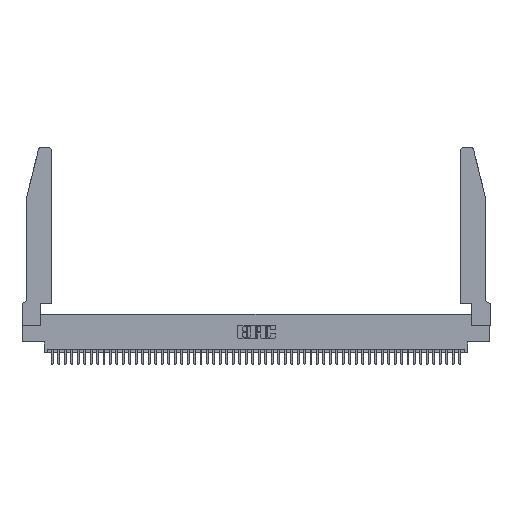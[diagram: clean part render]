
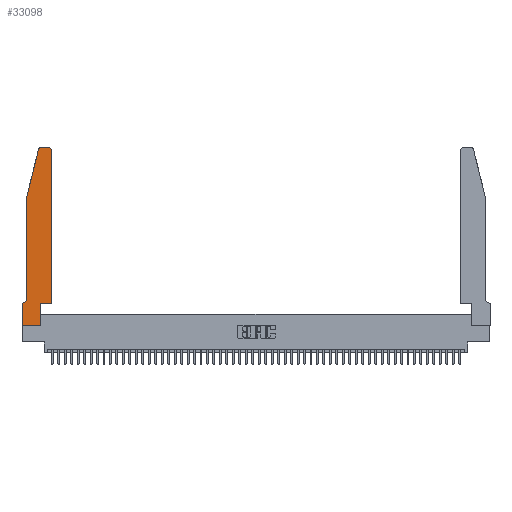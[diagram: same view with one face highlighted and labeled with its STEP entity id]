
A CAD part, top view. The second image highlights one B-rep face of the part: STEP entity #33098.
In plain terms, the highlighted planar face has unit normal (0, 0, 1).
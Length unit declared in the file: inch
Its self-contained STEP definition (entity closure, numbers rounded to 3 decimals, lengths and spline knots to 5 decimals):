
#779 = CARTESIAN_POINT ( 'NONE',  ( 0.4505, 0.35, 0.37 ) ) ;
#1848 = VECTOR ( 'NONE', #27411, 39.37008 ) ;
#1959 = EDGE_CURVE ( 'NONE', #48809, #43908, #16436, .T. ) ;
#2131 = DIRECTION ( 'NONE',  ( 1., 0., 0. ) ) ;
#2975 = ORIENTED_EDGE ( 'NONE', *, *, #28512, .T. ) ;
#3312 = CARTESIAN_POINT ( 'NONE',  ( 0., 0., 0.37 ) ) ;
#3450 = EDGE_CURVE ( 'NONE', #4753, #48809, #9399, .T. ) ;
#3521 = CARTESIAN_POINT ( 'NONE',  ( 0.0755, 2., 0.37 ) ) ;
#4753 = VERTEX_POINT ( 'NONE', #40390 ) ;
#4841 = CARTESIAN_POINT ( 'NONE',  ( 0.0755, 2., 0.37 ) ) ;
#5191 = LINE ( 'NONE', #779, #24251 ) ;
#6237 = EDGE_CURVE ( 'NONE', #11173, #46021, #50809, .T. ) ;
#6411 = VECTOR ( 'NONE', #9913, 39.37008 ) ;
#7217 = EDGE_CURVE ( 'NONE', #46886, #4753, #5191, .T. ) ;
#8631 = EDGE_CURVE ( 'NONE', #9656, #9747, #49717, .T. ) ;
#9015 = ORIENTED_EDGE ( 'NONE', *, *, #6237, .T. ) ;
#9399 = LINE ( 'NONE', #51511, #1848 ) ;
#9656 = VERTEX_POINT ( 'NONE', #24666 ) ;
#9747 = VERTEX_POINT ( 'NONE', #34577 ) ;
#9913 = DIRECTION ( 'NONE',  ( -1., 0., 0. ) ) ;
#10000 = CARTESIAN_POINT ( 'NONE',  ( 0.284, 2.72, 0.37 ) ) ;
#10002 = CARTESIAN_POINT ( 'NONE',  ( 0., 0.35, 0.37 ) ) ;
#11173 = VERTEX_POINT ( 'NONE', #37242 ) ;
#12496 = VECTOR ( 'NONE', #22220, 39.37008 ) ;
#13555 = ORIENTED_EDGE ( 'NONE', *, *, #1959, .T. ) ;
#14165 = DIRECTION ( 'NONE',  ( 1., 0., 0. ) ) ;
#15088 = ORIENTED_EDGE ( 'NONE', *, *, #28215, .T. ) ;
#15127 = ORIENTED_EDGE ( 'NONE', *, *, #3450, .T. ) ;
#16436 = CIRCLE ( 'NONE', #22639, 0.03 ) ;
#16842 = DIRECTION ( 'NONE',  ( 1., 0., 0. ) ) ;
#18253 = PLANE ( 'NONE',  #43515 ) ;
#18299 = VECTOR ( 'NONE', #2131, 39.37008 ) ;
#19898 = ORIENTED_EDGE ( 'NONE', *, *, #36210, .T. ) ;
#20077 = CARTESIAN_POINT ( 'NONE',  ( 0.2865, 0., 0.37 ) ) ;
#21431 = CARTESIAN_POINT ( 'NONE',  ( 0.4505, 2.72, 0.37 ) ) ;
#22161 = DIRECTION ( 'NONE',  ( 0., 0., 1. ) ) ;
#22216 = DIRECTION ( 'NONE',  ( 1., 0., 0. ) ) ;
#22220 = DIRECTION ( 'NONE',  ( 0., -1., 0. ) ) ;
#22243 = DIRECTION ( 'NONE',  ( -1., 0., 0. ) ) ;
#22639 = AXIS2_PLACEMENT_3D ( 'NONE', #30525, #38760, #26486 ) ;
#22997 = VECTOR ( 'NONE', #37019, 39.37008 ) ;
#23405 = DIRECTION ( 'NONE',  ( 0., -1., 0. ) ) ;
#23525 = LINE ( 'NONE', #3521, #24795 ) ;
#23817 = AXIS2_PLACEMENT_3D ( 'NONE', #10000, #38092, #22216 ) ;
#24251 = VECTOR ( 'NONE', #16842, 39.37008 ) ;
#24666 = CARTESIAN_POINT ( 'NONE',  ( 0.284, 2.75, 0.37 ) ) ;
#24795 = VECTOR ( 'NONE', #23405, 39.37008 ) ;
#25742 = CARTESIAN_POINT ( 'NONE',  ( 0., 0.35, 0.37 ) ) ;
#25931 = ORIENTED_EDGE ( 'NONE', *, *, #41141, .T. ) ;
#26433 = CARTESIAN_POINT ( 'NONE',  ( 0., 0., 0.37 ) ) ;
#26486 = DIRECTION ( 'NONE',  ( 1., 0., 0. ) ) ;
#26749 = DIRECTION ( 'NONE',  ( -1., 0., 0. ) ) ;
#26889 = EDGE_CURVE ( 'NONE', #9747, #51867, #27565, .T. ) ;
#27031 = VECTOR ( 'NONE', #37364, 39.37008 ) ;
#27411 = DIRECTION ( 'NONE',  ( 0., 1., 0. ) ) ;
#27565 = LINE ( 'NONE', #4841, #22997 ) ;
#28215 = EDGE_CURVE ( 'NONE', #43908, #9656, #31769, .T. ) ;
#28512 = EDGE_CURVE ( 'NONE', #51867, #11173, #23525, .T. ) ;
#30525 = CARTESIAN_POINT ( 'NONE',  ( 0.4205, 2.72, 0.37 ) ) ;
#30794 = ORIENTED_EDGE ( 'NONE', *, *, #8631, .T. ) ;
#30974 = LINE ( 'NONE', #26433, #18299 ) ;
#30993 = CARTESIAN_POINT ( 'NONE',  ( 0.4205, 2.75, 0.37 ) ) ;
#31046 = VERTEX_POINT ( 'NONE', #10002 ) ;
#31369 = FACE_OUTER_BOUND ( 'NONE', #48985, .T. ) ;
#31769 = LINE ( 'NONE', #37659, #6411 ) ;
#31829 = EDGE_CURVE ( 'NONE', #46021, #31046, #50353, .T. ) ;
#32724 = VECTOR ( 'NONE', #26749, 39.37008 ) ;
#33098 = ADVANCED_FACE ( 'NONE', ( #31369 ), #18253, .T. ) ;
#34577 = CARTESIAN_POINT ( 'NONE',  ( 0.25487, 2.72718, 0.37 ) ) ;
#35024 = CARTESIAN_POINT ( 'NONE',  ( 0.2865, 0.35, 0.37 ) ) ;
#36210 = EDGE_CURVE ( 'NONE', #37652, #44412, #30974, .T. ) ;
#37019 = DIRECTION ( 'NONE',  ( -0.239, -0.971, 0. ) ) ;
#37242 = CARTESIAN_POINT ( 'NONE',  ( 0.0755, 0.42, 0.37 ) ) ;
#37364 = DIRECTION ( 'NONE',  ( 0., 1., 0. ) ) ;
#37652 = VERTEX_POINT ( 'NONE', #3312 ) ;
#37659 = CARTESIAN_POINT ( 'NONE',  ( 0.2605, 2.75, 0.37 ) ) ;
#37694 = LINE ( 'NONE', #41916, #27031 ) ;
#38092 = DIRECTION ( 'NONE',  ( 0., 0., 1. ) ) ;
#38760 = DIRECTION ( 'NONE',  ( 0., 0., 1. ) ) ;
#39749 = EDGE_CURVE ( 'NONE', #44412, #46886, #37694, .T. ) ;
#40390 = CARTESIAN_POINT ( 'NONE',  ( 0.4505, 0.35, 0.37 ) ) ;
#40639 = AXIS2_PLACEMENT_3D ( 'NONE', #42349, #50805, #22243 ) ;
#41141 = EDGE_CURVE ( 'NONE', #31046, #37652, #51054, .T. ) ;
#41795 = CARTESIAN_POINT ( 'NONE',  ( 0.0755, 2., 0.37 ) ) ;
#41916 = CARTESIAN_POINT ( 'NONE',  ( 0.2865, 0.35, 0.37 ) ) ;
#42221 = CARTESIAN_POINT ( 'NONE',  ( 0.0755, 0.35, 0.37 ) ) ;
#42333 = ORIENTED_EDGE ( 'NONE', *, *, #39749, .T. ) ;
#42349 = CARTESIAN_POINT ( 'NONE',  ( 0.0055, 0.42, 0.37 ) ) ;
#43515 = AXIS2_PLACEMENT_3D ( 'NONE', #25742, #22161, #14165 ) ;
#43908 = VERTEX_POINT ( 'NONE', #30993 ) ;
#44412 = VERTEX_POINT ( 'NONE', #20077 ) ;
#45842 = CARTESIAN_POINT ( 'NONE',  ( 0.0055, 0.35, 0.37 ) ) ;
#46021 = VERTEX_POINT ( 'NONE', #45842 ) ;
#46691 = ORIENTED_EDGE ( 'NONE', *, *, #31829, .T. ) ;
#46886 = VERTEX_POINT ( 'NONE', #35024 ) ;
#46901 = ORIENTED_EDGE ( 'NONE', *, *, #26889, .T. ) ;
#47793 = ORIENTED_EDGE ( 'NONE', *, *, #7217, .T. ) ;
#48809 = VERTEX_POINT ( 'NONE', #21431 ) ;
#48985 = EDGE_LOOP ( 'NONE', ( #15088, #30794, #46901, #2975, #9015, #46691, #25931, #19898, #42333, #47793, #15127, #13555 ) ) ;
#49717 = CIRCLE ( 'NONE', #23817, 0.03 ) ;
#49911 = CARTESIAN_POINT ( 'NONE',  ( 0., 0., 0.37 ) ) ;
#50353 = LINE ( 'NONE', #42221, #32724 ) ;
#50805 = DIRECTION ( 'NONE',  ( 0., 0., -1. ) ) ;
#50809 = CIRCLE ( 'NONE', #40639, 0.07 ) ;
#51054 = LINE ( 'NONE', #49911, #12496 ) ;
#51511 = CARTESIAN_POINT ( 'NONE',  ( 0.4505, 0.35, 0.37 ) ) ;
#51867 = VERTEX_POINT ( 'NONE', #41795 ) ;
